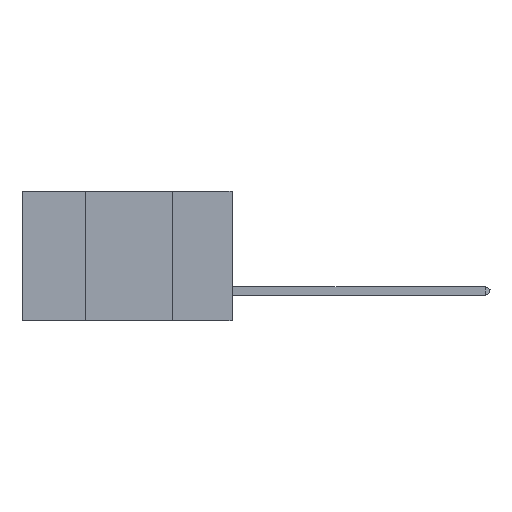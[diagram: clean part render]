
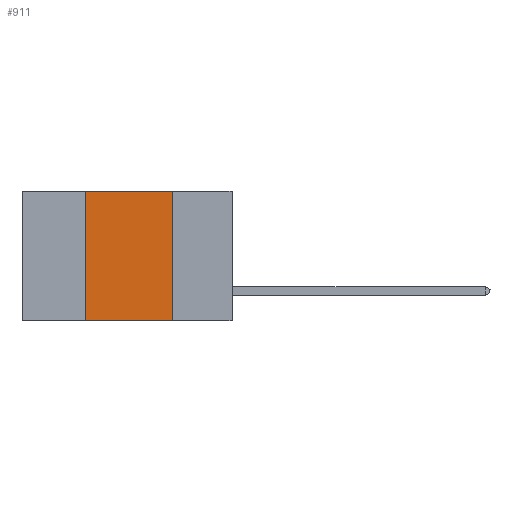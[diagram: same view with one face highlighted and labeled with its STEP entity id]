
A CAD part, left-side view. The second image highlights one B-rep face of the part: STEP entity #911.
In plain terms, the highlighted planar face has unit normal (-1, 0, 0).
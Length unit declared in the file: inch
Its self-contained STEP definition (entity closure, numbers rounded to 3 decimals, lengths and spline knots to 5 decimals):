
#264 = ORIENTED_EDGE ( 'NONE', *, *, #31543, .F. ) ;
#553 = DIRECTION ( 'NONE',  ( 0., 0., -1. ) ) ;
#911 = ADVANCED_FACE ( 'NONE', ( #17495 ), #3113, .F. ) ;
#1062 = CARTESIAN_POINT ( 'NONE',  ( 0., 0.42, -0.37 ) ) ;
#1222 = DIRECTION ( 'NONE',  ( 0., -1., 0. ) ) ;
#1837 = CARTESIAN_POINT ( 'NONE',  ( 0., 0.42, 0. ) ) ;
#2856 = LINE ( 'NONE', #35909, #13533 ) ;
#3113 = PLANE ( 'NONE',  #13843 ) ;
#3291 = VERTEX_POINT ( 'NONE', #1062 ) ;
#4397 = LINE ( 'NONE', #35551, #18303 ) ;
#7182 = VERTEX_POINT ( 'NONE', #29245 ) ;
#7376 = ORIENTED_EDGE ( 'NONE', *, *, #24111, .F. ) ;
#13526 = VERTEX_POINT ( 'NONE', #30354 ) ;
#13533 = VECTOR ( 'NONE', #24548, 39.37008 ) ;
#13843 = AXIS2_PLACEMENT_3D ( 'NONE', #27006, #23847, #553 ) ;
#17495 = FACE_OUTER_BOUND ( 'NONE', #36728, .T. ) ;
#18303 = VECTOR ( 'NONE', #1222, 39.37008 ) ;
#20907 = DIRECTION ( 'NONE',  ( 0., -1., 0. ) ) ;
#20966 = VERTEX_POINT ( 'NONE', #37142 ) ;
#21342 = LINE ( 'NONE', #1837, #22768 ) ;
#22242 = ORIENTED_EDGE ( 'NONE', *, *, #36305, .F. ) ;
#22768 = VECTOR ( 'NONE', #30142, 39.37008 ) ;
#23847 = DIRECTION ( 'NONE',  ( 1., 0., 0. ) ) ;
#24111 = EDGE_CURVE ( 'NONE', #3291, #7182, #21342, .T. ) ;
#24124 = LINE ( 'NONE', #26035, #33297 ) ;
#24548 = DIRECTION ( 'NONE',  ( 0., 0., -1. ) ) ;
#26035 = CARTESIAN_POINT ( 'NONE',  ( 0., 0.6, -0.37 ) ) ;
#26411 = ORIENTED_EDGE ( 'NONE', *, *, #37031, .T. ) ;
#27006 = CARTESIAN_POINT ( 'NONE',  ( 0., 0.6, 0. ) ) ;
#29245 = CARTESIAN_POINT ( 'NONE',  ( 0., 0.42, 0. ) ) ;
#30142 = DIRECTION ( 'NONE',  ( 0., 0., 1. ) ) ;
#30354 = CARTESIAN_POINT ( 'NONE',  ( 0., 0.17, 0. ) ) ;
#31543 = EDGE_CURVE ( 'NONE', #7182, #13526, #4397, .T. ) ;
#33297 = VECTOR ( 'NONE', #20907, 39.37008 ) ;
#35551 = CARTESIAN_POINT ( 'NONE',  ( 0., 0.6, 0. ) ) ;
#35909 = CARTESIAN_POINT ( 'NONE',  ( 0., 0.17, 0. ) ) ;
#36305 = EDGE_CURVE ( 'NONE', #13526, #20966, #2856, .T. ) ;
#36728 = EDGE_LOOP ( 'NONE', ( #22242, #264, #7376, #26411 ) ) ;
#37031 = EDGE_CURVE ( 'NONE', #3291, #20966, #24124, .T. ) ;
#37142 = CARTESIAN_POINT ( 'NONE',  ( 0., 0.17, -0.37 ) ) ;
